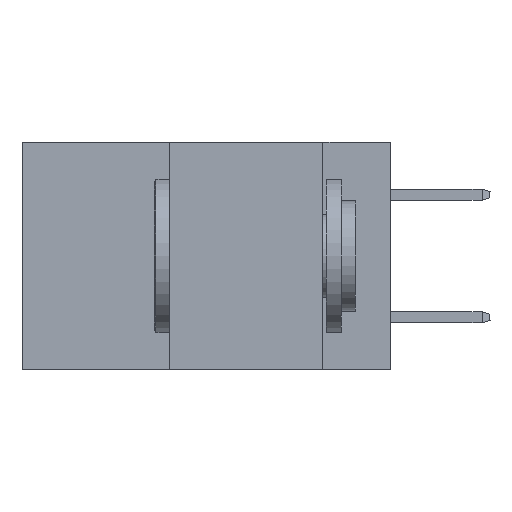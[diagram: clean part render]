
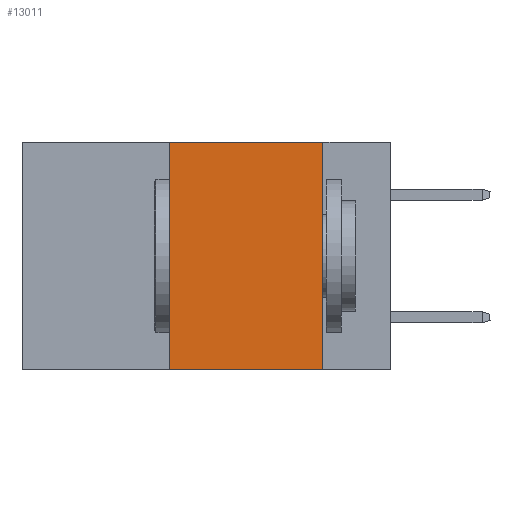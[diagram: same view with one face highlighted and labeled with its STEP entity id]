
A CAD part, left-side view. The second image highlights one B-rep face of the part: STEP entity #13011.
In plain terms, the highlighted planar face has unit normal (-1, 0, 0).
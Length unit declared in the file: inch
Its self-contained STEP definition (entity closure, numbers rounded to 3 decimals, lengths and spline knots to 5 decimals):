
#1659 = VECTOR ( 'NONE', #21576, 39.37008 ) ;
#2782 = LINE ( 'NONE', #27625, #4606 ) ;
#2886 = VERTEX_POINT ( 'NONE', #22580 ) ;
#4606 = VECTOR ( 'NONE', #18574, 39.37008 ) ;
#4964 = PLANE ( 'NONE',  #20440 ) ;
#5755 = LINE ( 'NONE', #33851, #20343 ) ;
#5790 = LINE ( 'NONE', #21829, #24977 ) ;
#6831 = EDGE_CURVE ( 'NONE', #15963, #22622, #5790, .T. ) ;
#7050 = EDGE_CURVE ( 'NONE', #2886, #16738, #5755, .T. ) ;
#8092 = EDGE_CURVE ( 'NONE', #2886, #15963, #30373, .T. ) ;
#8129 = CARTESIAN_POINT ( 'NONE',  ( 0., 0.6, 0. ) ) ;
#9154 = CARTESIAN_POINT ( 'NONE',  ( 0., 0.11, -0.37 ) ) ;
#13011 = ADVANCED_FACE ( 'NONE', ( #23487 ), #4964, .F. ) ;
#13736 = DIRECTION ( 'NONE',  ( 0., 0., -1. ) ) ;
#15963 = VERTEX_POINT ( 'NONE', #29762 ) ;
#16738 = VERTEX_POINT ( 'NONE', #9154 ) ;
#17137 = ORIENTED_EDGE ( 'NONE', *, *, #7050, .T. ) ;
#18574 = DIRECTION ( 'NONE',  ( 0., 0., -1. ) ) ;
#20034 = CARTESIAN_POINT ( 'NONE',  ( 0., 0.11, 0. ) ) ;
#20343 = VECTOR ( 'NONE', #36882, 39.37008 ) ;
#20440 = AXIS2_PLACEMENT_3D ( 'NONE', #8129, #28292, #13736 ) ;
#21576 = DIRECTION ( 'NONE',  ( 0., 0., 1. ) ) ;
#21829 = CARTESIAN_POINT ( 'NONE',  ( 0., 0.6, 0. ) ) ;
#22580 = CARTESIAN_POINT ( 'NONE',  ( 0., 0.36, -0.37 ) ) ;
#22622 = VERTEX_POINT ( 'NONE', #20034 ) ;
#23487 = FACE_OUTER_BOUND ( 'NONE', #37255, .T. ) ;
#24293 = ORIENTED_EDGE ( 'NONE', *, *, #8092, .F. ) ;
#24977 = VECTOR ( 'NONE', #33346, 39.37008 ) ;
#26909 = ORIENTED_EDGE ( 'NONE', *, *, #6831, .F. ) ;
#27341 = CARTESIAN_POINT ( 'NONE',  ( 0., 0.36, 0. ) ) ;
#27625 = CARTESIAN_POINT ( 'NONE',  ( 0., 0.11, 0. ) ) ;
#28292 = DIRECTION ( 'NONE',  ( 1., 0., 0. ) ) ;
#29762 = CARTESIAN_POINT ( 'NONE',  ( 0., 0.36, 0. ) ) ;
#30373 = LINE ( 'NONE', #27341, #1659 ) ;
#30956 = EDGE_CURVE ( 'NONE', #22622, #16738, #2782, .T. ) ;
#31666 = ORIENTED_EDGE ( 'NONE', *, *, #30956, .F. ) ;
#33346 = DIRECTION ( 'NONE',  ( 0., -1., 0. ) ) ;
#33851 = CARTESIAN_POINT ( 'NONE',  ( 0., 0.6, -0.37 ) ) ;
#36882 = DIRECTION ( 'NONE',  ( 0., -1., 0. ) ) ;
#37255 = EDGE_LOOP ( 'NONE', ( #31666, #26909, #24293, #17137 ) ) ;
